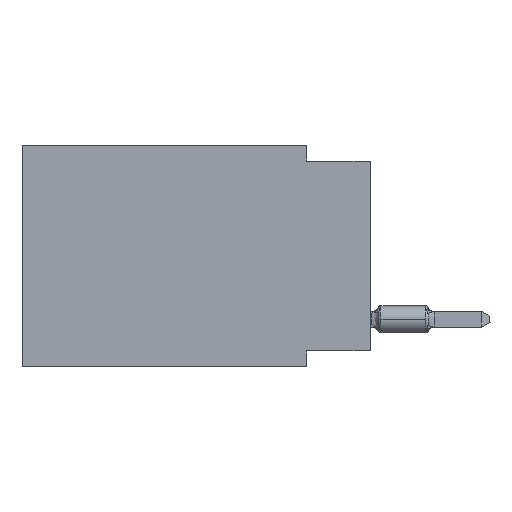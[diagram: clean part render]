
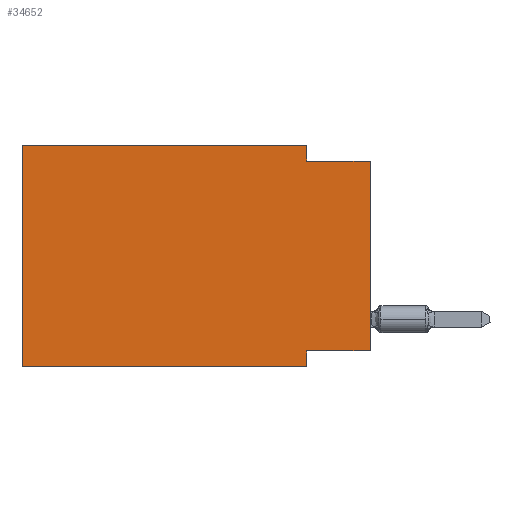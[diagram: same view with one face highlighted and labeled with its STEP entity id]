
A CAD part, left-side view. The second image highlights one B-rep face of the part: STEP entity #34652.
In plain terms, the highlighted planar face has unit normal (-1, 0, 0).
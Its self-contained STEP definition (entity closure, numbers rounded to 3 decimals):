
#825 = DIRECTION ( 'NONE',  ( 0., -1., 0. ) ) ;
#865 = DIRECTION ( 'NONE',  ( 0., 1., 0. ) ) ;
#2761 = VECTOR ( 'NONE', #14635, 1000. ) ;
#4536 = LINE ( 'NONE', #23542, #18163 ) ;
#5227 = DIRECTION ( 'NONE',  ( 0., 0., -1. ) ) ;
#5326 = CARTESIAN_POINT ( 'NONE',  ( 0., 13.97, 0. ) ) ;
#6298 = ORIENTED_EDGE ( 'NONE', *, *, #29358, .T. ) ;
#6523 = ORIENTED_EDGE ( 'NONE', *, *, #30920, .F. ) ;
#7017 = CARTESIAN_POINT ( 'NONE',  ( 0., 0., -8.255 ) ) ;
#8085 = VECTOR ( 'NONE', #33365, 1000. ) ;
#8141 = VERTEX_POINT ( 'NONE', #26713 ) ;
#8318 = VERTEX_POINT ( 'NONE', #30418 ) ;
#8407 = EDGE_CURVE ( 'NONE', #8141, #32193, #34442, .T. ) ;
#8924 = CARTESIAN_POINT ( 'NONE',  ( 0., 0., 0. ) ) ;
#9775 = CARTESIAN_POINT ( 'NONE',  ( 0., 13.97, 0. ) ) ;
#10505 = EDGE_CURVE ( 'NONE', #31811, #24544, #11852, .T. ) ;
#11310 = ORIENTED_EDGE ( 'NONE', *, *, #28399, .F. ) ;
#11354 = EDGE_CURVE ( 'NONE', #31811, #8318, #22071, .T. ) ;
#11655 = VERTEX_POINT ( 'NONE', #23899 ) ;
#11852 = LINE ( 'NONE', #16352, #17608 ) ;
#13606 = CARTESIAN_POINT ( 'NONE',  ( 0., 2.54, -8.255 ) ) ;
#14635 = DIRECTION ( 'NONE',  ( 0., -1., 0. ) ) ;
#15251 = VECTOR ( 'NONE', #23264, 1000. ) ;
#15669 = EDGE_CURVE ( 'NONE', #11655, #8318, #16943, .T. ) ;
#16158 = DIRECTION ( 'NONE',  ( 1., 0., 0. ) ) ;
#16352 = CARTESIAN_POINT ( 'NONE',  ( 0., 0., -8.255 ) ) ;
#16943 = LINE ( 'NONE', #25294, #2761 ) ;
#17608 = VECTOR ( 'NONE', #865, 1000. ) ;
#17656 = VECTOR ( 'NONE', #27591, 1000. ) ;
#18163 = VECTOR ( 'NONE', #18385, 1000. ) ;
#18385 = DIRECTION ( 'NONE',  ( 0., 0., -1. ) ) ;
#18627 = CARTESIAN_POINT ( 'NONE',  ( 0., 2.54, 0. ) ) ;
#18824 = PLANE ( 'NONE',  #25429 ) ;
#18873 = ORIENTED_EDGE ( 'NONE', *, *, #26550, .F. ) ;
#19376 = VERTEX_POINT ( 'NONE', #21523 ) ;
#20006 = EDGE_LOOP ( 'NONE', ( #30202, #34049, #11310, #18873, #34400, #6298, #6523, #32811 ) ) ;
#20034 = CARTESIAN_POINT ( 'NONE',  ( 0., 13.97, 0. ) ) ;
#20111 = CARTESIAN_POINT ( 'NONE',  ( 0., 13.97, 0. ) ) ;
#21523 = CARTESIAN_POINT ( 'NONE',  ( 0., 2.54, -8.89 ) ) ;
#22071 = LINE ( 'NONE', #8924, #17656 ) ;
#22357 = LINE ( 'NONE', #20034, #8085 ) ;
#23264 = DIRECTION ( 'NONE',  ( 0., 0., 1. ) ) ;
#23542 = CARTESIAN_POINT ( 'NONE',  ( 0., 2.54, 0. ) ) ;
#23899 = CARTESIAN_POINT ( 'NONE',  ( 0., 2.54, -0.635 ) ) ;
#24544 = VERTEX_POINT ( 'NONE', #13606 ) ;
#24571 = LINE ( 'NONE', #32927, #32361 ) ;
#25139 = LINE ( 'NONE', #30985, #32387 ) ;
#25294 = CARTESIAN_POINT ( 'NONE',  ( 0., 0., -0.635 ) ) ;
#25429 = AXIS2_PLACEMENT_3D ( 'NONE', #5326, #16158, #27000 ) ;
#26550 = EDGE_CURVE ( 'NONE', #32193, #31578, #22357, .T. ) ;
#26713 = CARTESIAN_POINT ( 'NONE',  ( 0., 13.97, -8.89 ) ) ;
#27000 = DIRECTION ( 'NONE',  ( 0., 0., -1. ) ) ;
#27591 = DIRECTION ( 'NONE',  ( 0., 0., 1. ) ) ;
#28399 = EDGE_CURVE ( 'NONE', #31578, #11655, #4536, .T. ) ;
#29358 = EDGE_CURVE ( 'NONE', #8141, #19376, #25139, .T. ) ;
#30202 = ORIENTED_EDGE ( 'NONE', *, *, #11354, .T. ) ;
#30418 = CARTESIAN_POINT ( 'NONE',  ( 0., 0., -0.635 ) ) ;
#30920 = EDGE_CURVE ( 'NONE', #24544, #19376, #24571, .T. ) ;
#30985 = CARTESIAN_POINT ( 'NONE',  ( 0., 13.97, -8.89 ) ) ;
#31578 = VERTEX_POINT ( 'NONE', #18627 ) ;
#31811 = VERTEX_POINT ( 'NONE', #7017 ) ;
#32142 = FACE_OUTER_BOUND ( 'NONE', #20006, .T. ) ;
#32193 = VERTEX_POINT ( 'NONE', #20111 ) ;
#32361 = VECTOR ( 'NONE', #5227, 1000. ) ;
#32387 = VECTOR ( 'NONE', #825, 1000. ) ;
#32811 = ORIENTED_EDGE ( 'NONE', *, *, #10505, .F. ) ;
#32927 = CARTESIAN_POINT ( 'NONE',  ( 0., 2.54, -8.89 ) ) ;
#33365 = DIRECTION ( 'NONE',  ( 0., -1., 0. ) ) ;
#34049 = ORIENTED_EDGE ( 'NONE', *, *, #15669, .F. ) ;
#34400 = ORIENTED_EDGE ( 'NONE', *, *, #8407, .F. ) ;
#34442 = LINE ( 'NONE', #9775, #15251 ) ;
#34652 = ADVANCED_FACE ( 'NONE', ( #32142 ), #18824, .F. ) ;
